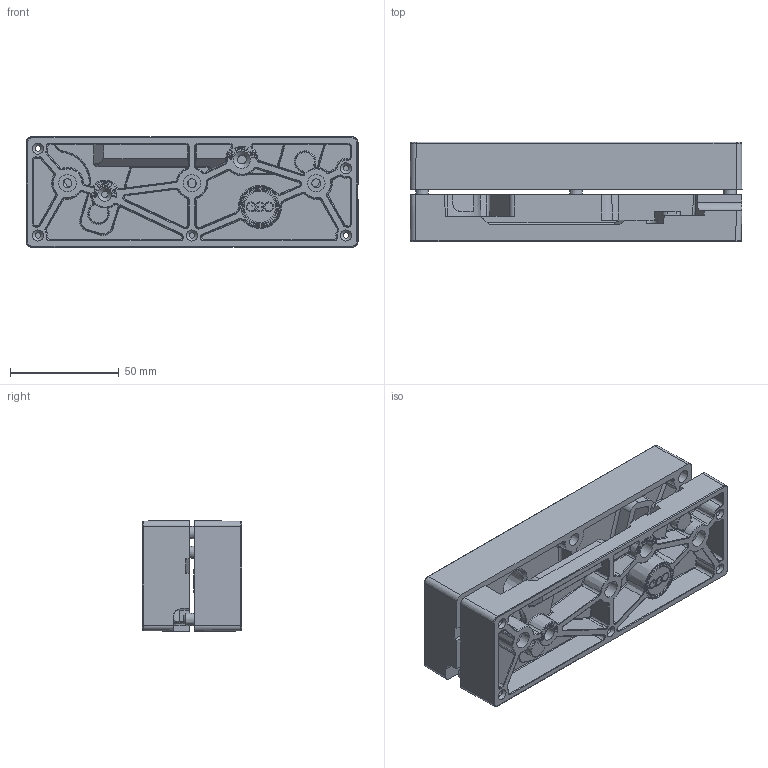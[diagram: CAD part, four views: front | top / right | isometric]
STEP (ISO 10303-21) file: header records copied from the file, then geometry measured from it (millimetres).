
FILE_DESCRIPTION(/* description */ ('Alibre Inc.'),/* implementation_level */ '2;1');
FILE_NAME(/* name */ 'G80 FIXTURE POLYMER REV E.step',/* time_stamp */ '2025-10-30T03:21:27-05:00',/* author */ (''),/* organization */ (''),/* preprocessor_version */ 'ST-DEVELOPER v20.1',/* originating_system */ 'Autodesk Translation Framework v14.17.0.0',/* authorisation */ '');
FILE_SCHEMA (('AUTOMOTIVE_DESIGN { 1 0 10303 214 3 1 1 }'));
Products named in the file (2): G80 FIXTURE IM RIGHT SIDE REV E v1; G80 FIXTURE IM LEFT SIDE REV E v1
Assembly tree (1 placements, depth 2):
  G80 FIXTURE IM RIGHT SIDE REV E v1
    G80 FIXTURE IM LEFT SIDE REV E v1
Bounding box: 152.49 x 45.6 x 50.86 mm (x, y, z)
Volume: 139459.1 mm3; surface area: 83529.1 mm2
Topology: 2 solids, 2 shells, 2586 faces, 6388 edges, 3892 vertices
Faces by surface type: bspline 900, plane 840, cylinder 479, torus 145, cone 139, sphere 83
Full cylindrical faces by diameter (mm): 2.54 x10, 3 x4, 3.048 x2, 4.039 x2, 4.064 x6, 6.35 x2, 7.938 x2, 8.001 x3, 17.403 x2
Entity records: 146792 total; most frequent: CARTESIAN_POINT 89834, ORIENTED_EDGE 12694, DIRECTION 10351, EDGE_CURVE 6347, VERTEX_POINT 3889, AXIS2_PLACEMENT_3D 3748, LINE 2855, VECTOR 2855
